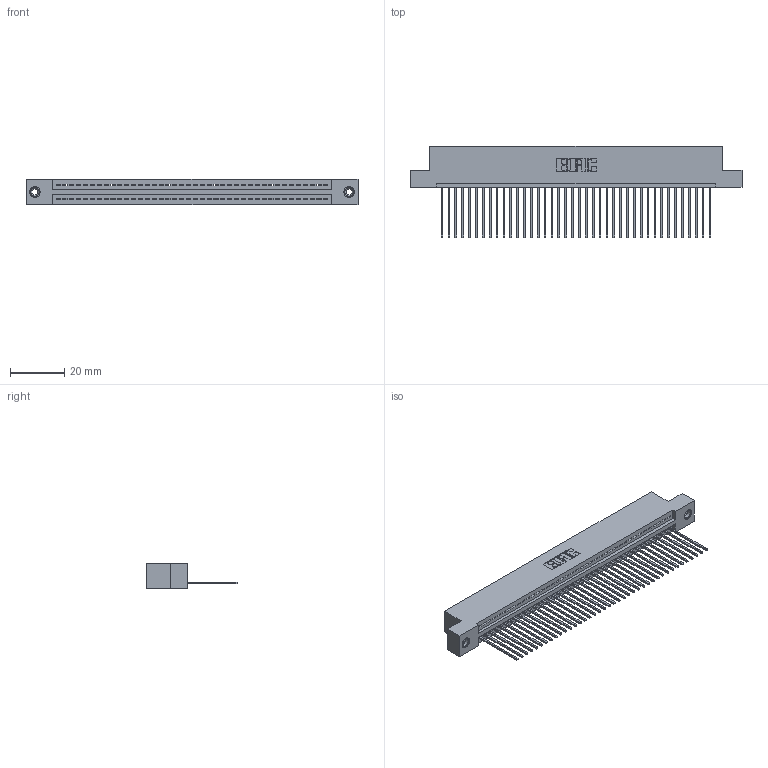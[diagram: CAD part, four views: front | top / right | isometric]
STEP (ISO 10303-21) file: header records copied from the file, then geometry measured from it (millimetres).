
FILE_DESCRIPTION (( 'STEP AP203' ), '1' );
FILE_NAME ('395-040-541-108.STEP', '2019-10-22T05:22:45', ( '' ), ( '' ), 'SwSTEP 2.0', 'SolidWorks 2016', '' );
FILE_SCHEMA (( 'CONFIG_CONTROL_DESIGN' ));
Length unit declared in the file: inch
Products named in the file (4): 345 Part_Flush Mounting Lugs - 0.156 Dia-TI; 395-040-541-108; 345-250-001_345-250-003-102; 345-292-001_345-293-141
Assembly tree (43 placements, depth 2):
  395-040-541-108
    345 Part_Flush Mounting Lugs - 0.156 Dia-TI
    345-292-001_345-293-141  x40
    345-250-001_345-250-003-102  x2
Bounding box: 122.81 x 33.96 x 9.4 mm (x, y, z)
Volume: 11773.6 mm3; surface area: 16414.7 mm2
Topology: 43 solids, 43 shells, 2506 faces, 7517 edges, 4950 vertices
Faces by surface type: plane 1712, cylinder 778, cone 12, torus 4
Entity records: 31578 total; most frequent: CARTESIAN_POINT 5451, ORIENTED_EDGE 5418, DIRECTION 4791, EDGE_CURVE 2709, LINE 2397, VECTOR 2397, VERTEX_POINT 1800, AXIS2_PLACEMENT_3D 1197
